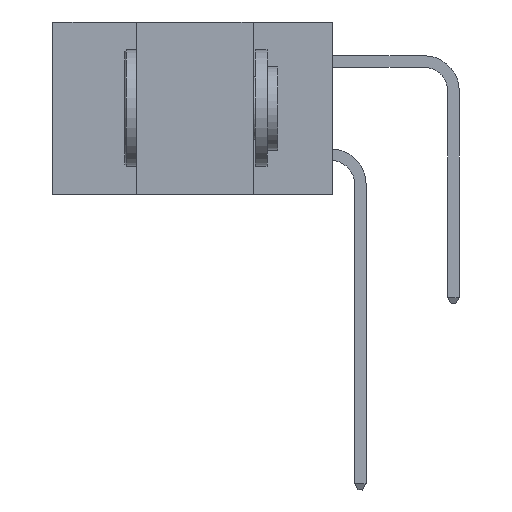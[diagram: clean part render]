
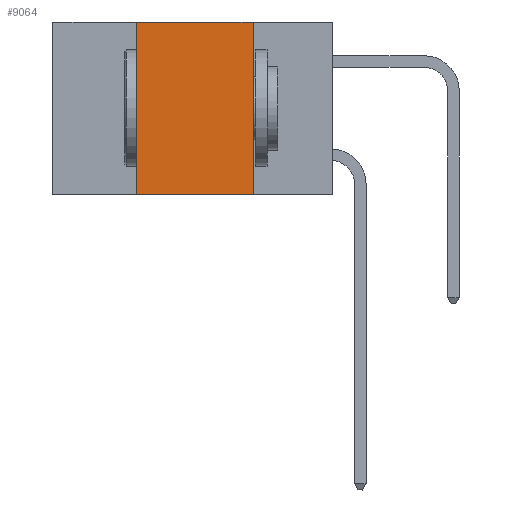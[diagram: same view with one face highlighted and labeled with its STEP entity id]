
A CAD part, left-side view. The second image highlights one B-rep face of the part: STEP entity #9064.
In plain terms, the highlighted planar face has unit normal (-1, 0, 0).
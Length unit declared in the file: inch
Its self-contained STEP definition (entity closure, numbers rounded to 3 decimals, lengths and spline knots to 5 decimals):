
#248 = CARTESIAN_POINT ( 'NONE',  ( 0., 0.6, 0. ) ) ;
#683 = ORIENTED_EDGE ( 'NONE', *, *, #2670, .F. ) ;
#766 = DIRECTION ( 'NONE',  ( 0., 0., -1. ) ) ;
#1583 = CARTESIAN_POINT ( 'NONE',  ( 0., 0.17, -0.37 ) ) ;
#2147 = VECTOR ( 'NONE', #8771, 39.37008 ) ;
#2259 = CARTESIAN_POINT ( 'NONE',  ( 0., 0.6, 0. ) ) ;
#2659 = CARTESIAN_POINT ( 'NONE',  ( 0., 0.17, -0.37 ) ) ;
#2670 = EDGE_CURVE ( 'NONE', #7903, #6484, #5309, .T. ) ;
#2764 = VECTOR ( 'NONE', #3274, 39.37008 ) ;
#3264 = CARTESIAN_POINT ( 'NONE',  ( 0., 0.42, -0.37 ) ) ;
#3274 = DIRECTION ( 'NONE',  ( 0., -1., 0. ) ) ;
#3984 = DIRECTION ( 'NONE',  ( 1., 0., 0. ) ) ;
#4096 = EDGE_CURVE ( 'NONE', #7903, #6407, #4899, .T. ) ;
#4841 = FACE_OUTER_BOUND ( 'NONE', #7935, .T. ) ;
#4899 = LINE ( 'NONE', #10623, #2147 ) ;
#5309 = LINE ( 'NONE', #3264, #10343 ) ;
#6099 = VERTEX_POINT ( 'NONE', #6701 ) ;
#6407 = VERTEX_POINT ( 'NONE', #1583 ) ;
#6484 = VERTEX_POINT ( 'NONE', #7322 ) ;
#6701 = CARTESIAN_POINT ( 'NONE',  ( 0., 0.17, 0. ) ) ;
#6984 = DIRECTION ( 'NONE',  ( 0., 0., 1. ) ) ;
#7103 = AXIS2_PLACEMENT_3D ( 'NONE', #248, #3984, #7760 ) ;
#7322 = CARTESIAN_POINT ( 'NONE',  ( 0., 0.42, 0. ) ) ;
#7361 = EDGE_CURVE ( 'NONE', #6099, #6407, #11021, .T. ) ;
#7760 = DIRECTION ( 'NONE',  ( 0., 0., -1. ) ) ;
#7807 = CARTESIAN_POINT ( 'NONE',  ( 0., 0.42, -0.37 ) ) ;
#7903 = VERTEX_POINT ( 'NONE', #7807 ) ;
#7935 = EDGE_LOOP ( 'NONE', ( #11123, #9540, #683, #9208 ) ) ;
#7990 = EDGE_CURVE ( 'NONE', #6484, #6099, #8763, .T. ) ;
#8667 = PLANE ( 'NONE',  #7103 ) ;
#8763 = LINE ( 'NONE', #2259, #2764 ) ;
#8771 = DIRECTION ( 'NONE',  ( 0., -1., 0. ) ) ;
#9064 = ADVANCED_FACE ( 'NONE', ( #4841 ), #8667, .F. ) ;
#9208 = ORIENTED_EDGE ( 'NONE', *, *, #4096, .T. ) ;
#9214 = VECTOR ( 'NONE', #766, 39.37008 ) ;
#9540 = ORIENTED_EDGE ( 'NONE', *, *, #7990, .F. ) ;
#10343 = VECTOR ( 'NONE', #6984, 39.37008 ) ;
#10623 = CARTESIAN_POINT ( 'NONE',  ( 0., 0.6, -0.37 ) ) ;
#11021 = LINE ( 'NONE', #2659, #9214 ) ;
#11123 = ORIENTED_EDGE ( 'NONE', *, *, #7361, .F. ) ;
